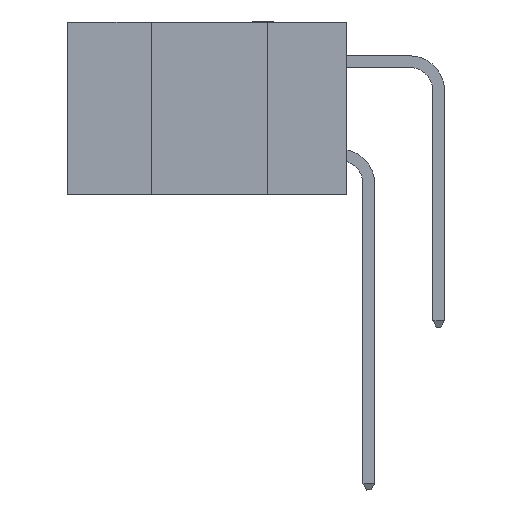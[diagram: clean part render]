
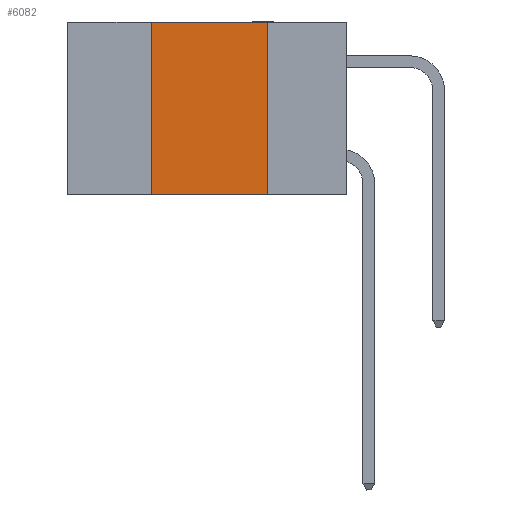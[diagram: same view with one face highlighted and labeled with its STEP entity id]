
A CAD part, left-side view. The second image highlights one B-rep face of the part: STEP entity #6082.
In plain terms, the highlighted planar face has unit normal (-1, 0, 0).
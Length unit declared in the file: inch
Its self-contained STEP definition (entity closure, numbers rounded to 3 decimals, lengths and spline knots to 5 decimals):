
#551 = VECTOR ( 'NONE', #25417, 39.37008 ) ;
#649 = CARTESIAN_POINT ( 'NONE',  ( 0., 0.17, -0.37 ) ) ;
#2584 = CARTESIAN_POINT ( 'NONE',  ( 0., 0.17, 0. ) ) ;
#3742 = VERTEX_POINT ( 'NONE', #13273 ) ;
#4326 = CARTESIAN_POINT ( 'NONE',  ( 0., 0.6, 0. ) ) ;
#6082 = ADVANCED_FACE ( 'NONE', ( #21852 ), #21739, .F. ) ;
#6086 = EDGE_CURVE ( 'NONE', #32118, #16115, #11494, .T. ) ;
#7823 = DIRECTION ( 'NONE',  ( 0., 0., -1. ) ) ;
#8409 = LINE ( 'NONE', #2584, #15535 ) ;
#9894 = LINE ( 'NONE', #42627, #551 ) ;
#10391 = CARTESIAN_POINT ( 'NONE',  ( 0., 0.42, -0.37 ) ) ;
#11494 = LINE ( 'NONE', #15500, #20791 ) ;
#13273 = CARTESIAN_POINT ( 'NONE',  ( 0., 0.42, 0. ) ) ;
#14110 = EDGE_CURVE ( 'NONE', #34844, #16115, #8409, .T. ) ;
#14203 = ORIENTED_EDGE ( 'NONE', *, *, #29619, .F. ) ;
#14366 = AXIS2_PLACEMENT_3D ( 'NONE', #4326, #28723, #7823 ) ;
#15500 = CARTESIAN_POINT ( 'NONE',  ( 0., 0.6, -0.37 ) ) ;
#15535 = VECTOR ( 'NONE', #27156, 39.37008 ) ;
#16115 = VERTEX_POINT ( 'NONE', #649 ) ;
#20791 = VECTOR ( 'NONE', #39723, 39.37008 ) ;
#21739 = PLANE ( 'NONE',  #14366 ) ;
#21852 = FACE_OUTER_BOUND ( 'NONE', #33913, .T. ) ;
#24366 = DIRECTION ( 'NONE',  ( 0., -1., 0. ) ) ;
#25417 = DIRECTION ( 'NONE',  ( 0., 0., 1. ) ) ;
#25925 = LINE ( 'NONE', #41547, #43223 ) ;
#27156 = DIRECTION ( 'NONE',  ( 0., 0., -1. ) ) ;
#28723 = DIRECTION ( 'NONE',  ( 1., 0., 0. ) ) ;
#29401 = ORIENTED_EDGE ( 'NONE', *, *, #6086, .T. ) ;
#29619 = EDGE_CURVE ( 'NONE', #32118, #3742, #9894, .T. ) ;
#32118 = VERTEX_POINT ( 'NONE', #10391 ) ;
#33913 = EDGE_LOOP ( 'NONE', ( #35395, #44016, #14203, #29401 ) ) ;
#34844 = VERTEX_POINT ( 'NONE', #39587 ) ;
#35395 = ORIENTED_EDGE ( 'NONE', *, *, #14110, .F. ) ;
#39587 = CARTESIAN_POINT ( 'NONE',  ( 0., 0.17, 0. ) ) ;
#39723 = DIRECTION ( 'NONE',  ( 0., -1., 0. ) ) ;
#41547 = CARTESIAN_POINT ( 'NONE',  ( 0., 0.6, 0. ) ) ;
#42627 = CARTESIAN_POINT ( 'NONE',  ( 0., 0.42, 0. ) ) ;
#43223 = VECTOR ( 'NONE', #24366, 39.37008 ) ;
#43459 = EDGE_CURVE ( 'NONE', #3742, #34844, #25925, .T. ) ;
#44016 = ORIENTED_EDGE ( 'NONE', *, *, #43459, .F. ) ;
